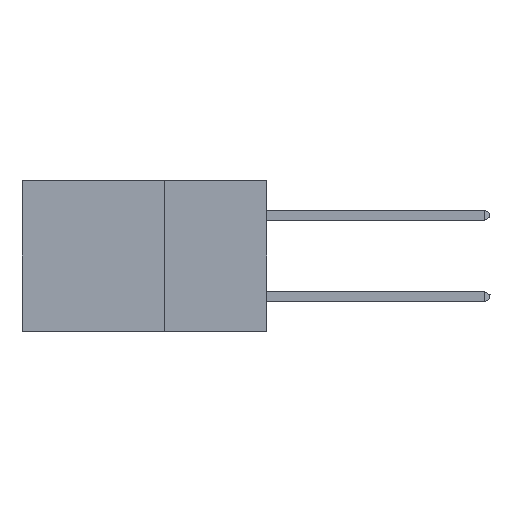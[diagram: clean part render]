
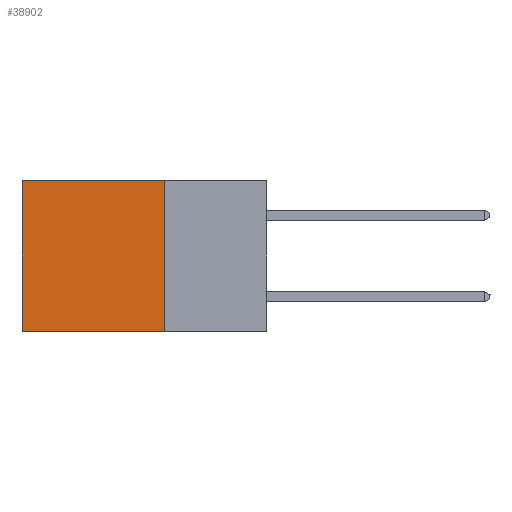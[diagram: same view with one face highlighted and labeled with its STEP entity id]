
A CAD part, left-side view. The second image highlights one B-rep face of the part: STEP entity #38902.
In plain terms, the highlighted planar face has unit normal (-1, 0, 0).
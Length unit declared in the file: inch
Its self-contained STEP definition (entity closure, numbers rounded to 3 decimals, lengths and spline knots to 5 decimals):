
#1468 = VECTOR ( 'NONE', #29736, 39.37008 ) ;
#2552 = LINE ( 'NONE', #24955, #14144 ) ;
#2750 = FACE_OUTER_BOUND ( 'NONE', #11545, .T. ) ;
#3064 = VERTEX_POINT ( 'NONE', #22623 ) ;
#4450 = CARTESIAN_POINT ( 'NONE',  ( 0.2875, 0.25, 0. ) ) ;
#4619 = VERTEX_POINT ( 'NONE', #34264 ) ;
#5329 = VERTEX_POINT ( 'NONE', #4450 ) ;
#5719 = ORIENTED_EDGE ( 'NONE', *, *, #36592, .F. ) ;
#5806 = PLANE ( 'NONE',  #33230 ) ;
#6368 = CARTESIAN_POINT ( 'NONE',  ( 0.2875, 0.25, 0. ) ) ;
#9584 = EDGE_CURVE ( 'NONE', #4619, #31476, #20399, .T. ) ;
#11545 = EDGE_LOOP ( 'NONE', ( #22546, #5719, #17434, #38079 ) ) ;
#14144 = VECTOR ( 'NONE', #25179, 39.37008 ) ;
#16185 = DIRECTION ( 'NONE',  ( 0., 1., 0. ) ) ;
#16308 = VECTOR ( 'NONE', #36655, 39.37008 ) ;
#17434 = ORIENTED_EDGE ( 'NONE', *, *, #31103, .F. ) ;
#19518 = EDGE_CURVE ( 'NONE', #5329, #4619, #23502, .T. ) ;
#19938 = CARTESIAN_POINT ( 'NONE',  ( 0.2875, 0.25, 0. ) ) ;
#20399 = LINE ( 'NONE', #20986, #16308 ) ;
#20986 = CARTESIAN_POINT ( 'NONE',  ( 0.2875, 0.6, 0. ) ) ;
#22546 = ORIENTED_EDGE ( 'NONE', *, *, #9584, .T. ) ;
#22623 = CARTESIAN_POINT ( 'NONE',  ( 0.2875, 0.25, -0.37 ) ) ;
#23502 = LINE ( 'NONE', #32714, #40824 ) ;
#24955 = CARTESIAN_POINT ( 'NONE',  ( 0.2875, 0.25, -0.37 ) ) ;
#25179 = DIRECTION ( 'NONE',  ( 0., 1., 0. ) ) ;
#25892 = LINE ( 'NONE', #19938, #1468 ) ;
#28561 = DIRECTION ( 'NONE',  ( 1., 0., 0. ) ) ;
#29736 = DIRECTION ( 'NONE',  ( 0., 0., -1. ) ) ;
#31103 = EDGE_CURVE ( 'NONE', #5329, #3064, #25892, .T. ) ;
#31476 = VERTEX_POINT ( 'NONE', #37859 ) ;
#32714 = CARTESIAN_POINT ( 'NONE',  ( 0.2875, 0.25, 0. ) ) ;
#33230 = AXIS2_PLACEMENT_3D ( 'NONE', #6368, #28561, #35108 ) ;
#34264 = CARTESIAN_POINT ( 'NONE',  ( 0.2875, 0.6, 0. ) ) ;
#35108 = DIRECTION ( 'NONE',  ( 0., 0., -1. ) ) ;
#36592 = EDGE_CURVE ( 'NONE', #3064, #31476, #2552, .T. ) ;
#36655 = DIRECTION ( 'NONE',  ( 0., 0., -1. ) ) ;
#37859 = CARTESIAN_POINT ( 'NONE',  ( 0.2875, 0.6, -0.37 ) ) ;
#38079 = ORIENTED_EDGE ( 'NONE', *, *, #19518, .T. ) ;
#38902 = ADVANCED_FACE ( 'NONE', ( #2750 ), #5806, .F. ) ;
#40824 = VECTOR ( 'NONE', #16185, 39.37008 ) ;
